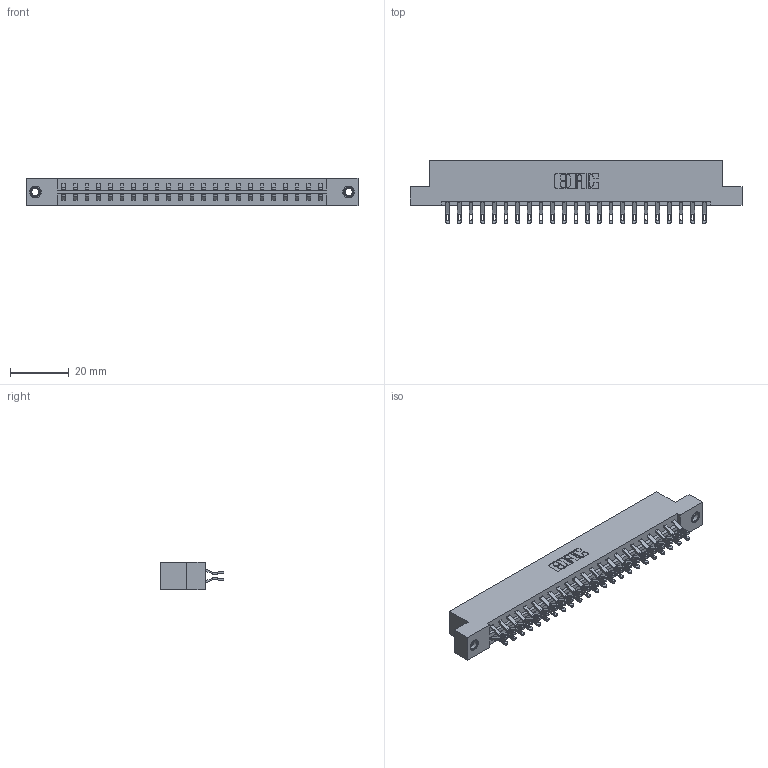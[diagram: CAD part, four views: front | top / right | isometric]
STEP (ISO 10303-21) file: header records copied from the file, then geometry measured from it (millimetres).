
FILE_DESCRIPTION (( 'STEP AP203' ), '1' );
FILE_NAME ('333-046-555-207.STEP', '2018-08-03T22:40:28', ( '' ), ( '' ), 'SwSTEP 2.0', 'SolidWorks 2016', '' );
FILE_SCHEMA (( 'CONFIG_CONTROL_DESIGN' ));
Length unit declared in the file: inch
Products named in the file (4): 333 Part_Flush - .156 Dia - TI; 345-292-001_555 Tail; 345-250-001_345-250-005-103; 333-046-555-207
Assembly tree (49 placements, depth 2):
  333-046-555-207
    333 Part_Flush - .156 Dia - TI
    345-292-001_555 Tail  x46
    345-250-001_345-250-005-103  x2
Bounding box: 112.67 x 21.47 x 9.4 mm (x, y, z)
Volume: 11445.6 mm3; surface area: 13860.5 mm2
Topology: 49 solids, 49 shells, 2842 faces, 8865 edges, 5902 vertices
Faces by surface type: plane 1666, cylinder 1160, cone 12, torus 4
Entity records: 18766 total; most frequent: CARTESIAN_POINT 3151, ORIENTED_EDGE 3050, DIRECTION 2727, EDGE_CURVE 1525, LINE 1357, VECTOR 1357, VERTEX_POINT 1012, AXIS2_PLACEMENT_3D 685
